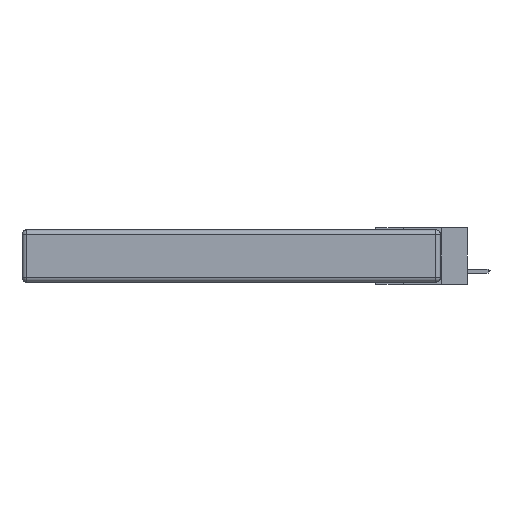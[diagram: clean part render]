
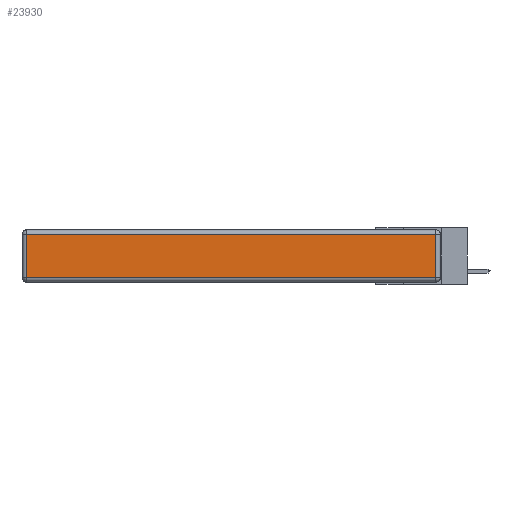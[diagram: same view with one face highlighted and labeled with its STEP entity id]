
A CAD part, left-side view. The second image highlights one B-rep face of the part: STEP entity #23930.
In plain terms, the highlighted planar face has unit normal (-1, 0, 0).
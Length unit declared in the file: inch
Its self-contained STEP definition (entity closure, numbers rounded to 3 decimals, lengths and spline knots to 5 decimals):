
#2221 = CARTESIAN_POINT ( 'NONE',  ( 0., 0., -0.343 ) ) ;
#2286 = AXIS2_PLACEMENT_3D ( 'NONE', #2221, #33328, #7663 ) ;
#4407 = VERTEX_POINT ( 'NONE', #6602 ) ;
#4659 = VECTOR ( 'NONE', #13962, 39.37008 ) ;
#6602 = CARTESIAN_POINT ( 'NONE',  ( 0., 2.72, -0.03 ) ) ;
#7124 = ORIENTED_EDGE ( 'NONE', *, *, #15178, .T. ) ;
#7663 = DIRECTION ( 'NONE',  ( 0., 0., 1. ) ) ;
#10136 = LINE ( 'NONE', #17647, #29878 ) ;
#10612 = VECTOR ( 'NONE', #15705, 39.37008 ) ;
#13755 = LINE ( 'NONE', #28830, #4659 ) ;
#13962 = DIRECTION ( 'NONE',  ( 0., 0., 1. ) ) ;
#15178 = EDGE_CURVE ( 'NONE', #4407, #26747, #10136, .T. ) ;
#15526 = LINE ( 'NONE', #21154, #10612 ) ;
#15705 = DIRECTION ( 'NONE',  ( 0., 1., 0. ) ) ;
#17531 = DIRECTION ( 'NONE',  ( 0., 0., -1. ) ) ;
#17647 = CARTESIAN_POINT ( 'NONE',  ( 0., 2.72, -0.343 ) ) ;
#19994 = EDGE_CURVE ( 'NONE', #31518, #23297, #13755, .T. ) ;
#20691 = PLANE ( 'NONE',  #2286 ) ;
#20779 = VECTOR ( 'NONE', #29306, 39.37008 ) ;
#20783 = FACE_OUTER_BOUND ( 'NONE', #26710, .T. ) ;
#21154 = CARTESIAN_POINT ( 'NONE',  ( 0., 2.75, -0.03 ) ) ;
#22348 = ORIENTED_EDGE ( 'NONE', *, *, #19994, .T. ) ;
#23166 = EDGE_CURVE ( 'NONE', #26747, #31518, #27753, .T. ) ;
#23297 = VERTEX_POINT ( 'NONE', #24025 ) ;
#23930 = ADVANCED_FACE ( 'NONE', ( #20783 ), #20691, .T. ) ;
#24025 = CARTESIAN_POINT ( 'NONE',  ( 0., 0.03, -0.03 ) ) ;
#24676 = ORIENTED_EDGE ( 'NONE', *, *, #32018, .T. ) ;
#25643 = CARTESIAN_POINT ( 'NONE',  ( 0., 2.72, -0.313 ) ) ;
#26700 = ORIENTED_EDGE ( 'NONE', *, *, #23166, .T. ) ;
#26710 = EDGE_LOOP ( 'NONE', ( #26700, #22348, #24676, #7124 ) ) ;
#26747 = VERTEX_POINT ( 'NONE', #25643 ) ;
#27052 = CARTESIAN_POINT ( 'NONE',  ( 0., 0.03, -0.313 ) ) ;
#27753 = LINE ( 'NONE', #29747, #20779 ) ;
#28830 = CARTESIAN_POINT ( 'NONE',  ( 0., 0.03, -0.343 ) ) ;
#29306 = DIRECTION ( 'NONE',  ( 0., -1., 0. ) ) ;
#29747 = CARTESIAN_POINT ( 'NONE',  ( 0., 0., -0.313 ) ) ;
#29878 = VECTOR ( 'NONE', #17531, 39.37008 ) ;
#31518 = VERTEX_POINT ( 'NONE', #27052 ) ;
#32018 = EDGE_CURVE ( 'NONE', #23297, #4407, #15526, .T. ) ;
#33328 = DIRECTION ( 'NONE',  ( -1., 0., 0. ) ) ;
